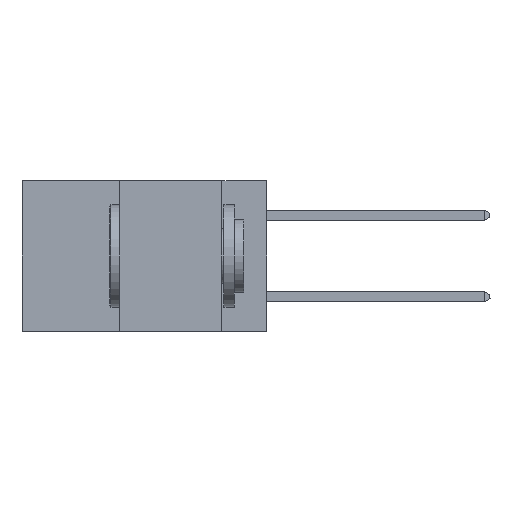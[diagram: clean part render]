
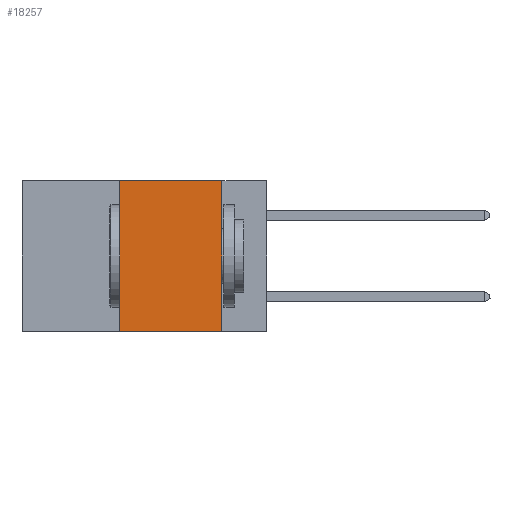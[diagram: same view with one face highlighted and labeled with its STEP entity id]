
A CAD part, left-side view. The second image highlights one B-rep face of the part: STEP entity #18257.
In plain terms, the highlighted planar face has unit normal (-1, 0, 0).
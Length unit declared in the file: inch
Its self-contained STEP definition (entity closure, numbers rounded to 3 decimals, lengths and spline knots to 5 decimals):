
#135 = ORIENTED_EDGE ( 'NONE', *, *, #17378, .F. ) ;
#949 = VERTEX_POINT ( 'NONE', #4172 ) ;
#1290 = DIRECTION ( 'NONE',  ( 0., 0., 1. ) ) ;
#2459 = EDGE_LOOP ( 'NONE', ( #15188, #135, #26592, #8492 ) ) ;
#2677 = DIRECTION ( 'NONE',  ( 1., 0., 0. ) ) ;
#3366 = LINE ( 'NONE', #9706, #4344 ) ;
#4123 = EDGE_CURVE ( 'NONE', #17551, #949, #6561, .T. ) ;
#4172 = CARTESIAN_POINT ( 'NONE',  ( 0., 0.11, -0.37 ) ) ;
#4173 = CARTESIAN_POINT ( 'NONE',  ( 0., 0.36, -0.37 ) ) ;
#4344 = VECTOR ( 'NONE', #1290, 39.37008 ) ;
#6308 = AXIS2_PLACEMENT_3D ( 'NONE', #23157, #2677, #25201 ) ;
#6561 = LINE ( 'NONE', #15191, #16892 ) ;
#7624 = DIRECTION ( 'NONE',  ( 0., -1., 0. ) ) ;
#8492 = ORIENTED_EDGE ( 'NONE', *, *, #4123, .T. ) ;
#9706 = CARTESIAN_POINT ( 'NONE',  ( 0., 0.36, 0. ) ) ;
#11964 = FACE_OUTER_BOUND ( 'NONE', #2459, .T. ) ;
#13461 = CARTESIAN_POINT ( 'NONE',  ( 0., 0.36, 0. ) ) ;
#14381 = VERTEX_POINT ( 'NONE', #13461 ) ;
#15188 = ORIENTED_EDGE ( 'NONE', *, *, #17272, .F. ) ;
#15191 = CARTESIAN_POINT ( 'NONE',  ( 0., 0.6, -0.37 ) ) ;
#15833 = CARTESIAN_POINT ( 'NONE',  ( 0., 0.11, 0. ) ) ;
#16014 = CARTESIAN_POINT ( 'NONE',  ( 0., 0.6, 0. ) ) ;
#16892 = VECTOR ( 'NONE', #25322, 39.37008 ) ;
#16910 = VECTOR ( 'NONE', #26236, 39.37008 ) ;
#17272 = EDGE_CURVE ( 'NONE', #19266, #949, #20091, .T. ) ;
#17378 = EDGE_CURVE ( 'NONE', #14381, #19266, #23979, .T. ) ;
#17551 = VERTEX_POINT ( 'NONE', #4173 ) ;
#18257 = ADVANCED_FACE ( 'NONE', ( #11964 ), #25372, .F. ) ;
#18478 = VECTOR ( 'NONE', #7624, 39.37008 ) ;
#19266 = VERTEX_POINT ( 'NONE', #15833 ) ;
#20091 = LINE ( 'NONE', #26335, #16910 ) ;
#23157 = CARTESIAN_POINT ( 'NONE',  ( 0., 0.6, 0. ) ) ;
#23979 = LINE ( 'NONE', #16014, #18478 ) ;
#25162 = EDGE_CURVE ( 'NONE', #17551, #14381, #3366, .T. ) ;
#25201 = DIRECTION ( 'NONE',  ( 0., 0., -1. ) ) ;
#25322 = DIRECTION ( 'NONE',  ( 0., -1., 0. ) ) ;
#25372 = PLANE ( 'NONE',  #6308 ) ;
#26236 = DIRECTION ( 'NONE',  ( 0., 0., -1. ) ) ;
#26335 = CARTESIAN_POINT ( 'NONE',  ( 0., 0.11, 0. ) ) ;
#26592 = ORIENTED_EDGE ( 'NONE', *, *, #25162, .F. ) ;
